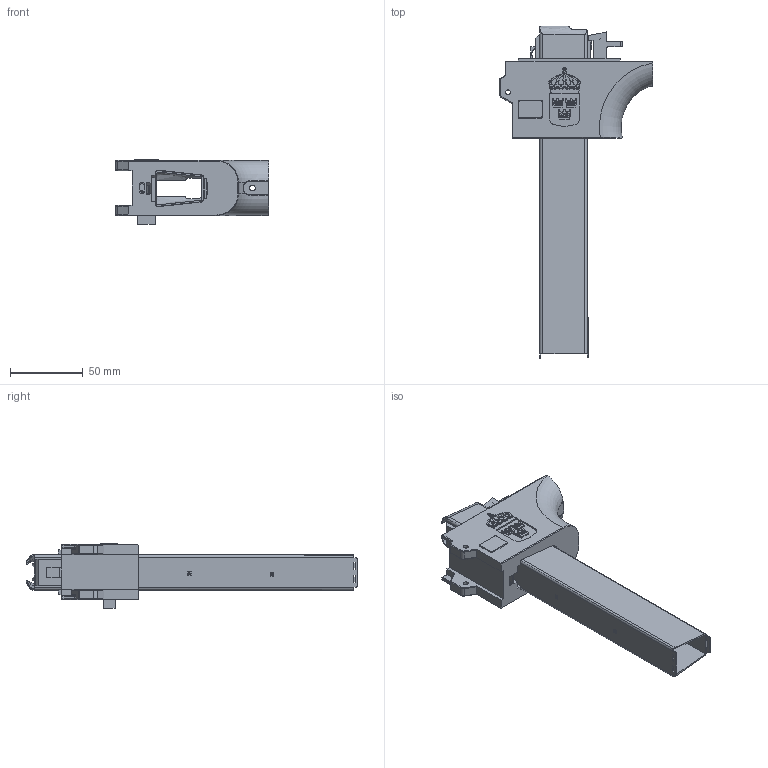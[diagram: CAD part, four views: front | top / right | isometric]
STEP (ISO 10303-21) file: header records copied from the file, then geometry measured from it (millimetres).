
FILE_DESCRIPTION(/* description */ (''),/* implementation_level */ '2;1');
FILE_NAME(/* name */ 'm45 assembly final.stp',/* time_stamp */ '2021-07-08T22:03:26+02:00',/* author */ (''),/* organization */ (''),/* preprocessor_version */ 'ST-DEVELOPER v15.2',/* originating_system */ 'Autodesk Translator Framework v2.0.0.5431',/* authorisation */ '');
FILE_SCHEMA (('AUTOMOTIVE_DESIGN { 1 0 10303 214 3 1 1 }'));
Length unit declared in the file: centimetre
Products named in the file (1): (Unsaved)
Bounding box: 105.51 x 228.73 x 44.5 mm (x, y, z)
Volume: 145599.1 mm3; surface area: 80090 mm2
Topology: 5 solids, 5 shells, 731 faces, 2036 edges, 1336 vertices
Faces by surface type: plane 357, bspline 281, cylinder 78, torus 8, sphere 4, cone 3
Full cylindrical faces by diameter (mm): 1.5 x2, 3 x1, 3.4 x2, 4 x1
Entity records: 28236 total; most frequent: CARTESIAN_POINT 11264, ORIENTED_EDGE 4048, DIRECTION 2543, EDGE_CURVE 2024, VERTEX_POINT 1336, LINE 1263, VECTOR 1263, EDGE_LOOP 794
